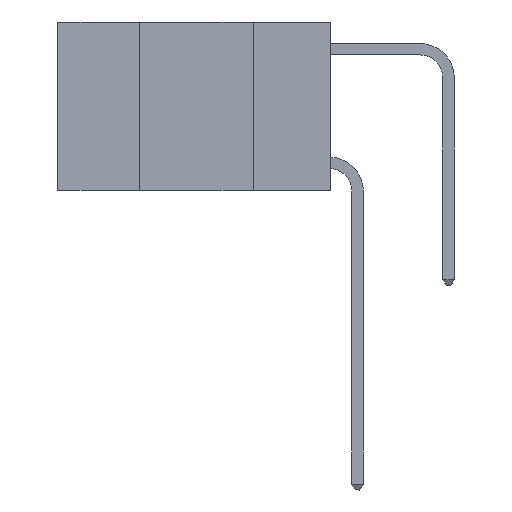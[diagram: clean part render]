
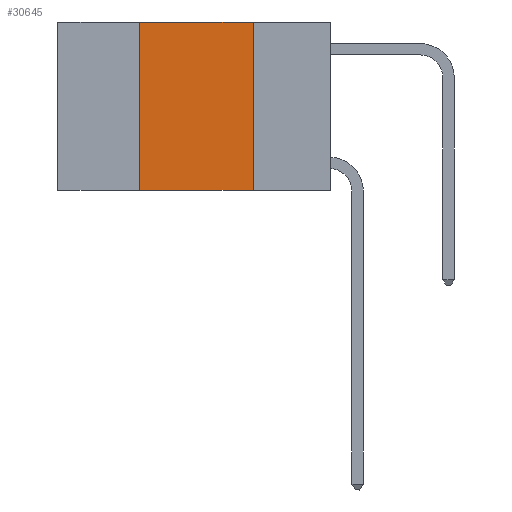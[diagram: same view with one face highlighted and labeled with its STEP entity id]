
A CAD part, left-side view. The second image highlights one B-rep face of the part: STEP entity #30645.
In plain terms, the highlighted planar face has unit normal (-1, 0, 0).
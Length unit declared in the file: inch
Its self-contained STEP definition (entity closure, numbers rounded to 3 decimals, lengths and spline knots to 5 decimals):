
#626 = AXIS2_PLACEMENT_3D ( 'NONE', #14847, #19652, #4523 ) ;
#1382 = VERTEX_POINT ( 'NONE', #8753 ) ;
#3695 = DIRECTION ( 'NONE',  ( 0., 0., 1. ) ) ;
#4372 = DIRECTION ( 'NONE',  ( 0., -1., 0. ) ) ;
#4523 = DIRECTION ( 'NONE',  ( 0., 0., -1. ) ) ;
#4864 = CARTESIAN_POINT ( 'NONE',  ( 0., 0.42, -0.37 ) ) ;
#7157 = EDGE_LOOP ( 'NONE', ( #12726, #23400, #21810, #17235 ) ) ;
#8753 = CARTESIAN_POINT ( 'NONE',  ( 0., 0.17, 0. ) ) ;
#9494 = VERTEX_POINT ( 'NONE', #17930 ) ;
#9587 = DIRECTION ( 'NONE',  ( 0., -1., 0. ) ) ;
#9657 = EDGE_CURVE ( 'NONE', #10494, #18589, #9821, .T. ) ;
#9821 = LINE ( 'NONE', #21812, #29333 ) ;
#10481 = DIRECTION ( 'NONE',  ( 0., 0., -1. ) ) ;
#10494 = VERTEX_POINT ( 'NONE', #4864 ) ;
#10537 = FACE_OUTER_BOUND ( 'NONE', #7157, .T. ) ;
#10900 = EDGE_CURVE ( 'NONE', #10494, #9494, #32831, .T. ) ;
#12251 = CARTESIAN_POINT ( 'NONE',  ( 0., 0.42, 0. ) ) ;
#12726 = ORIENTED_EDGE ( 'NONE', *, *, #31572, .F. ) ;
#13016 = CARTESIAN_POINT ( 'NONE',  ( 0., 0.17, 0. ) ) ;
#14847 = CARTESIAN_POINT ( 'NONE',  ( 0., 0.6, 0. ) ) ;
#17235 = ORIENTED_EDGE ( 'NONE', *, *, #10900, .T. ) ;
#17930 = CARTESIAN_POINT ( 'NONE',  ( 0., 0.17, -0.37 ) ) ;
#18589 = VERTEX_POINT ( 'NONE', #12251 ) ;
#19652 = DIRECTION ( 'NONE',  ( 1., 0., 0. ) ) ;
#20647 = CARTESIAN_POINT ( 'NONE',  ( 0., 0.6, -0.37 ) ) ;
#21810 = ORIENTED_EDGE ( 'NONE', *, *, #9657, .F. ) ;
#21812 = CARTESIAN_POINT ( 'NONE',  ( 0., 0.42, 0. ) ) ;
#23400 = ORIENTED_EDGE ( 'NONE', *, *, #31453, .F. ) ;
#24669 = PLANE ( 'NONE',  #626 ) ;
#24818 = VECTOR ( 'NONE', #9587, 39.37008 ) ;
#24869 = LINE ( 'NONE', #13016, #28869 ) ;
#26443 = LINE ( 'NONE', #27765, #30451 ) ;
#27765 = CARTESIAN_POINT ( 'NONE',  ( 0., 0.6, 0. ) ) ;
#28869 = VECTOR ( 'NONE', #10481, 39.37008 ) ;
#29333 = VECTOR ( 'NONE', #3695, 39.37008 ) ;
#30451 = VECTOR ( 'NONE', #4372, 39.37008 ) ;
#30645 = ADVANCED_FACE ( 'NONE', ( #10537 ), #24669, .F. ) ;
#31453 = EDGE_CURVE ( 'NONE', #18589, #1382, #26443, .T. ) ;
#31572 = EDGE_CURVE ( 'NONE', #1382, #9494, #24869, .T. ) ;
#32831 = LINE ( 'NONE', #20647, #24818 ) ;
